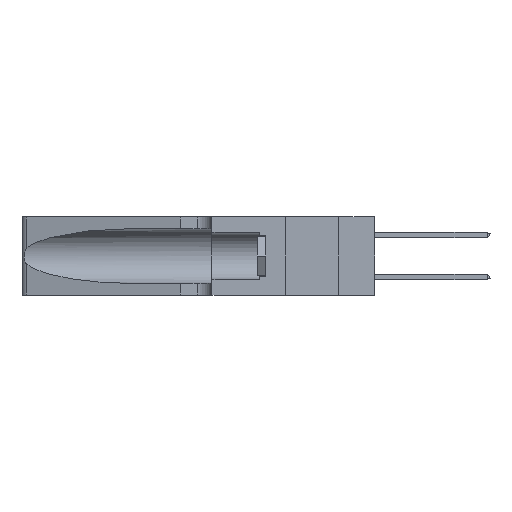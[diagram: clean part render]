
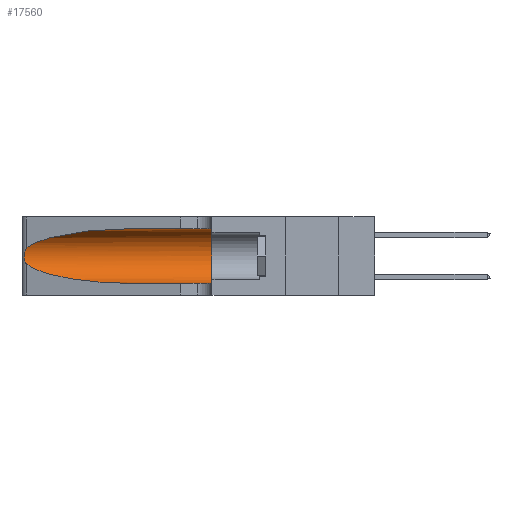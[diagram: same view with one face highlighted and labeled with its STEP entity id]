
A CAD part, left-side view. The second image highlights one B-rep face of the part: STEP entity #17560.
In plain terms, the highlighted cylindrical face has radius 3.308 mm (diameter 6.617 mm), a partial arc.
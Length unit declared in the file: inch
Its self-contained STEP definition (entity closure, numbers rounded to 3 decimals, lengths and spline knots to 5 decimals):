
#165 = AXIS2_PLACEMENT_3D ( 'NONE', #27909, #16404, #2936 ) ;
#622 = EDGE_CURVE ( 'NONE', #11621, #8102, #20696, .T. ) ;
#675 = VERTEX_POINT ( 'NONE', #26341 ) ;
#2235 = CARTESIAN_POINT ( 'NONE',  ( 0.1305, 0.72297, 0.05475 ) ) ;
#2514 = CARTESIAN_POINT ( 'NONE',  ( 0.25639, 1.23184, 0.21858 ) ) ;
#2607 = CARTESIAN_POINT ( 'NONE',  ( 0.25487, 1.22718, 0.14631 ) ) ;
#2936 = DIRECTION ( 'NONE',  ( 0., 0., -1. ) ) ;
#4903 = CARTESIAN_POINT ( 'NONE',  ( 0.25555, 1.22993, 0.14849 ) ) ;
#5787 = VERTEX_POINT ( 'NONE', #11514 ) ;
#6092 = CARTESIAN_POINT ( 'NONE',  ( 0.1305, 0.35, 0.185 ) ) ;
#6470 = VECTOR ( 'NONE', #11577, 39.37008 ) ;
#6718 = EDGE_CURVE ( 'NONE', #23423, #5787, #10951, .T. ) ;
#6896 = CARTESIAN_POINT ( 'NONE',  ( 0.1305, 0.35, 0.31525 ) ) ;
#6931 = CARTESIAN_POINT ( 'NONE',  ( 0.25639, 1.23186, 0.15144 ) ) ;
#7599 = CARTESIAN_POINT ( 'NONE',  ( 0.1305, 1.61858, 0.31525 ) ) ;
#7659 = ORIENTED_EDGE ( 'NONE', *, *, #28787, .F. ) ;
#7894 = CARTESIAN_POINT ( 'NONE',  ( 0.1305, 0.35, 0.05475 ) ) ;
#8102 = VERTEX_POINT ( 'NONE', #7894 ) ;
#8457 = CARTESIAN_POINT ( 'NONE',  ( 0.18966, 0.96281, 0.31525 ) ) ;
#8587 = CARTESIAN_POINT ( 'NONE',  ( 0.1305, 0.72297, 0.31525 ) ) ;
#8959 = ORIENTED_EDGE ( 'NONE', *, *, #6718, .T. ) ;
#10245 = CARTESIAN_POINT ( 'NONE',  ( 0.25487, 1.22718, 0.22369 ) ) ;
#10360 = EDGE_CURVE ( 'NONE', #5787, #675, #12192, .T. ) ;
#10951 =( BOUNDED_CURVE ( )  B_SPLINE_CURVE ( 3, ( #12220, #8457, #12934, #10245 ),
 .UNSPECIFIED., .F., .F. ) 
 B_SPLINE_CURVE_WITH_KNOTS ( ( 4, 4 ),
 ( 1.5708, 2.84003 ),
 .UNSPECIFIED. ) 
 CURVE ( )  GEOMETRIC_REPRESENTATION_ITEM ( )  RATIONAL_B_SPLINE_CURVE ( ( 1., 0.87, 0.87, 1. ) ) 
 REPRESENTATION_ITEM ( '' )  );
#11514 = CARTESIAN_POINT ( 'NONE',  ( 0.25487, 1.22718, 0.22369 ) ) ;
#11577 = DIRECTION ( 'NONE',  ( 0., -1., 0. ) ) ;
#11621 = VERTEX_POINT ( 'NONE', #25855 ) ;
#11669 = CARTESIAN_POINT ( 'NONE',  ( 0.26017, 1.23833, 0.17102 ) ) ;
#12134 = DIRECTION ( 'NONE',  ( 0., -1., 0. ) ) ;
#12192 = B_SPLINE_CURVE_WITH_KNOTS ( 'NONE', 3,
 ( #13409, #22625, #2514, #22999, #27379, #13769, #24907, #25282, #11669, #27579, #16296, #6931, #4903, #2607 ),
 .UNSPECIFIED., .F., .F.,
 ( 4, 2, 2, 2, 2, 2, 4 ),
 ( 0., 0.00027, 0.00053, 0.00107, 0.0016, 0.00187, 0.00214 ),
 .UNSPECIFIED. ) ;
#12217 = ORIENTED_EDGE ( 'NONE', *, *, #10360, .T. ) ;
#12220 = CARTESIAN_POINT ( 'NONE',  ( 0.1305, 0.72297, 0.31525 ) ) ;
#12934 = CARTESIAN_POINT ( 'NONE',  ( 0.2373, 1.15595, 0.28018 ) ) ;
#13406 = CARTESIAN_POINT ( 'NONE',  ( 0.18966, 0.96281, 0.05475 ) ) ;
#13409 = CARTESIAN_POINT ( 'NONE',  ( 0.25487, 1.22718, 0.22369 ) ) ;
#13591 = CARTESIAN_POINT ( 'NONE',  ( 0.25487, 1.22718, 0.14631 ) ) ;
#13769 = CARTESIAN_POINT ( 'NONE',  ( 0.26018, 1.23835, 0.19895 ) ) ;
#14851 = VERTEX_POINT ( 'NONE', #6896 ) ;
#15501 = CARTESIAN_POINT ( 'NONE',  ( 0.2373, 1.15595, 0.08982 ) ) ;
#16296 = CARTESIAN_POINT ( 'NONE',  ( 0.25789, 1.23486, 0.15765 ) ) ;
#16404 = DIRECTION ( 'NONE',  ( 0., -1., 0. ) ) ;
#17312 = EDGE_CURVE ( 'NONE', #675, #11621, #28986, .T. ) ;
#17316 = EDGE_LOOP ( 'NONE', ( #8959, #12217, #20543, #22635, #19659, #7659 ) ) ;
#17560 = ADVANCED_FACE ( 'NONE', ( #20288 ), #26302, .F. ) ;
#19659 = ORIENTED_EDGE ( 'NONE', *, *, #20402, .F. ) ;
#20288 = FACE_OUTER_BOUND ( 'NONE', #17316, .T. ) ;
#20402 = EDGE_CURVE ( 'NONE', #14851, #8102, #23227, .T. ) ;
#20541 = CARTESIAN_POINT ( 'NONE',  ( 0.1305, 1.61858, 0.05475 ) ) ;
#20543 = ORIENTED_EDGE ( 'NONE', *, *, #17312, .T. ) ;
#20696 = LINE ( 'NONE', #20541, #6470 ) ;
#22625 = CARTESIAN_POINT ( 'NONE',  ( 0.25555, 1.22994, 0.2215 ) ) ;
#22635 = ORIENTED_EDGE ( 'NONE', *, *, #622, .T. ) ;
#22999 = CARTESIAN_POINT ( 'NONE',  ( 0.25787, 1.23484, 0.2124 ) ) ;
#23227 = CIRCLE ( 'NONE', #29163, 0.13025 ) ;
#23423 = VERTEX_POINT ( 'NONE', #8587 ) ;
#24047 = LINE ( 'NONE', #7599, #28680 ) ;
#24907 = CARTESIAN_POINT ( 'NONE',  ( 0.26075, 1.23896, 0.19203 ) ) ;
#25282 = CARTESIAN_POINT ( 'NONE',  ( 0.26075, 1.23896, 0.178 ) ) ;
#25855 = CARTESIAN_POINT ( 'NONE',  ( 0.1305, 0.72297, 0.05475 ) ) ;
#26302 = CYLINDRICAL_SURFACE ( 'NONE', #165, 0.13025 ) ;
#26341 = CARTESIAN_POINT ( 'NONE',  ( 0.25487, 1.22718, 0.14631 ) ) ;
#26581 = DIRECTION ( 'NONE',  ( 0., 0., 1. ) ) ;
#27379 = CARTESIAN_POINT ( 'NONE',  ( 0.25854, 1.2359, 0.20912 ) ) ;
#27579 = CARTESIAN_POINT ( 'NONE',  ( 0.25856, 1.23593, 0.16098 ) ) ;
#27909 = CARTESIAN_POINT ( 'NONE',  ( 0.1305, 1.61858, 0.185 ) ) ;
#28557 = DIRECTION ( 'NONE',  ( 0., 1., 0. ) ) ;
#28680 = VECTOR ( 'NONE', #12134, 39.37008 ) ;
#28787 = EDGE_CURVE ( 'NONE', #23423, #14851, #24047, .T. ) ;
#28986 =( BOUNDED_CURVE ( )  B_SPLINE_CURVE ( 3, ( #13591, #15501, #13406, #2235 ),
 .UNSPECIFIED., .F., .F. ) 
 B_SPLINE_CURVE_WITH_KNOTS ( ( 4, 4 ),
 ( 3.44316, 4.71239 ),
 .UNSPECIFIED. ) 
 CURVE ( )  GEOMETRIC_REPRESENTATION_ITEM ( )  RATIONAL_B_SPLINE_CURVE ( ( 1., 0.87, 0.87, 1. ) ) 
 REPRESENTATION_ITEM ( '' )  );
#29163 = AXIS2_PLACEMENT_3D ( 'NONE', #6092, #28557, #26581 ) ;
